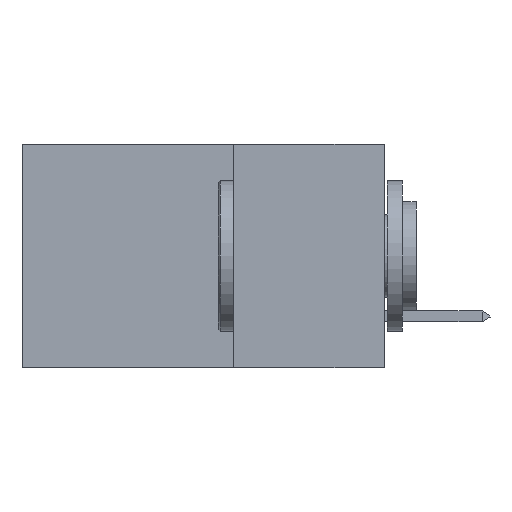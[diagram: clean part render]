
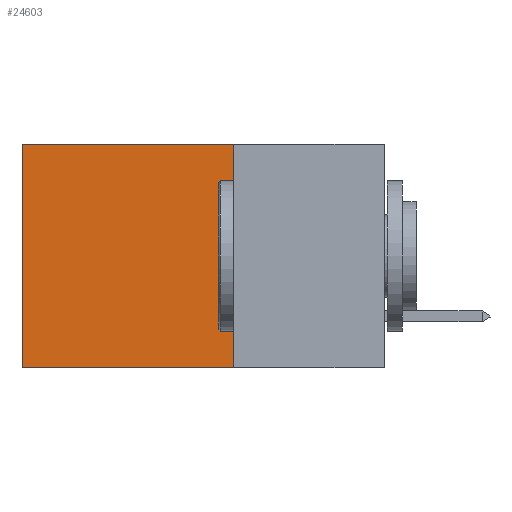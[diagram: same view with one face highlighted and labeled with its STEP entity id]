
A CAD part, left-side view. The second image highlights one B-rep face of the part: STEP entity #24603.
In plain terms, the highlighted planar face has unit normal (-1, 0, 0).
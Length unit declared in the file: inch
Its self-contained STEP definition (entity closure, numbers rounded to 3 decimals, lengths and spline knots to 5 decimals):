
#395 = EDGE_CURVE ( 'NONE', #17351, #4485, #27817, .T. ) ;
#1253 = DIRECTION ( 'NONE',  ( 0., 1., 0. ) ) ;
#1296 = FACE_OUTER_BOUND ( 'NONE', #20666, .T. ) ;
#1476 = DIRECTION ( 'NONE',  ( 0., 0., -1. ) ) ;
#1580 = PLANE ( 'NONE',  #18943 ) ;
#2233 = ORIENTED_EDGE ( 'NONE', *, *, #18727, .F. ) ;
#2939 = LINE ( 'NONE', #20735, #7244 ) ;
#4485 = VERTEX_POINT ( 'NONE', #24493 ) ;
#6606 = CARTESIAN_POINT ( 'NONE',  ( 0.2875, 0.25, 0. ) ) ;
#7244 = VECTOR ( 'NONE', #1253, 39.37008 ) ;
#11930 = CARTESIAN_POINT ( 'NONE',  ( 0.2875, 0.6, 0. ) ) ;
#12648 = DIRECTION ( 'NONE',  ( 0., 0., -1. ) ) ;
#13194 = VECTOR ( 'NONE', #25688, 39.37008 ) ;
#15292 = VECTOR ( 'NONE', #19920, 39.37008 ) ;
#16444 = VERTEX_POINT ( 'NONE', #23719 ) ;
#16546 = LINE ( 'NONE', #17459, #18094 ) ;
#16755 = ORIENTED_EDGE ( 'NONE', *, *, #27454, .F. ) ;
#17351 = VERTEX_POINT ( 'NONE', #27380 ) ;
#17459 = CARTESIAN_POINT ( 'NONE',  ( 0.2875, 0.25, 0. ) ) ;
#18094 = VECTOR ( 'NONE', #12648, 39.37008 ) ;
#18407 = VERTEX_POINT ( 'NONE', #31358 ) ;
#18727 = EDGE_CURVE ( 'NONE', #18407, #16444, #16546, .T. ) ;
#18943 = AXIS2_PLACEMENT_3D ( 'NONE', #6606, #24109, #1476 ) ;
#19792 = ORIENTED_EDGE ( 'NONE', *, *, #26880, .T. ) ;
#19920 = DIRECTION ( 'NONE',  ( 0., 0., -1. ) ) ;
#20633 = LINE ( 'NONE', #28401, #13194 ) ;
#20666 = EDGE_LOOP ( 'NONE', ( #29762, #16755, #2233, #19792 ) ) ;
#20735 = CARTESIAN_POINT ( 'NONE',  ( 0.2875, 0.25, -0.37 ) ) ;
#23719 = CARTESIAN_POINT ( 'NONE',  ( 0.2875, 0.25, -0.37 ) ) ;
#24109 = DIRECTION ( 'NONE',  ( 1., 0., 0. ) ) ;
#24493 = CARTESIAN_POINT ( 'NONE',  ( 0.2875, 0.6, -0.37 ) ) ;
#24603 = ADVANCED_FACE ( 'NONE', ( #1296 ), #1580, .F. ) ;
#25688 = DIRECTION ( 'NONE',  ( 0., 1., 0. ) ) ;
#26880 = EDGE_CURVE ( 'NONE', #18407, #17351, #20633, .T. ) ;
#27380 = CARTESIAN_POINT ( 'NONE',  ( 0.2875, 0.6, 0. ) ) ;
#27454 = EDGE_CURVE ( 'NONE', #16444, #4485, #2939, .T. ) ;
#27817 = LINE ( 'NONE', #11930, #15292 ) ;
#28401 = CARTESIAN_POINT ( 'NONE',  ( 0.2875, 0.25, 0. ) ) ;
#29762 = ORIENTED_EDGE ( 'NONE', *, *, #395, .T. ) ;
#31358 = CARTESIAN_POINT ( 'NONE',  ( 0.2875, 0.25, 0. ) ) ;
